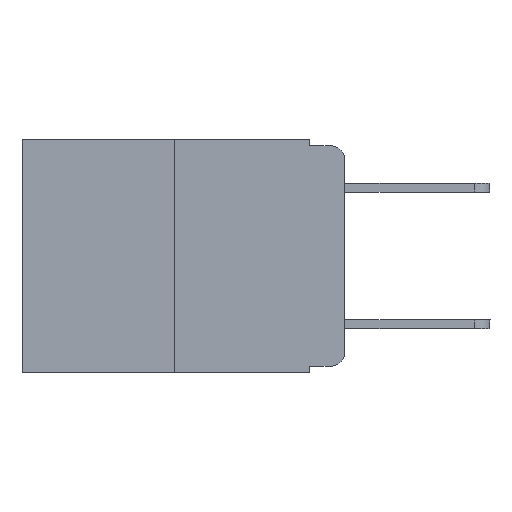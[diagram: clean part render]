
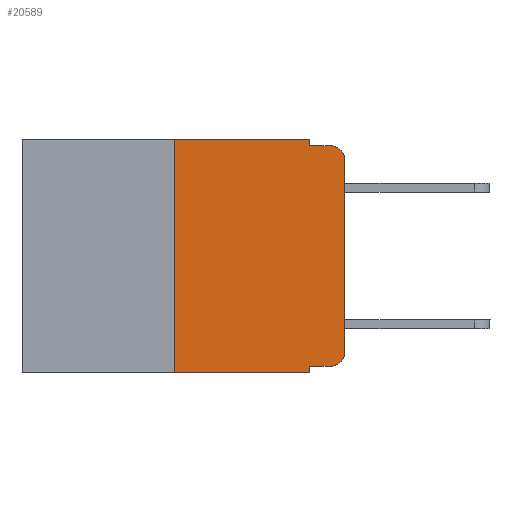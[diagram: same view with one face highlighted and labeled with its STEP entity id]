
A CAD part, left-side view. The second image highlights one B-rep face of the part: STEP entity #20589.
In plain terms, the highlighted planar face has unit normal (-1, 0, 0).
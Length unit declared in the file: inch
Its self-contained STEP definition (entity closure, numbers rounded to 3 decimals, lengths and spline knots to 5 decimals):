
#69 = DIRECTION ( 'NONE',  ( 0., 0., -1. ) ) ;
#441 = DIRECTION ( 'NONE',  ( 0., -1., 0. ) ) ;
#652 = EDGE_LOOP ( 'NONE', ( #15446, #8806, #4839, #7220, #18919, #14201, #16379, #14491, #13478, #13454 ) ) ;
#856 = CARTESIAN_POINT ( 'NONE',  ( 0., 0.473, 0. ) ) ;
#1182 = VERTEX_POINT ( 'NONE', #15359 ) ;
#1519 = VECTOR ( 'NONE', #8959, 39.37008 ) ;
#1958 = CARTESIAN_POINT ( 'NONE',  ( 0., 0.051, 0. ) ) ;
#2366 = VECTOR ( 'NONE', #7526, 39.37008 ) ;
#3283 = EDGE_CURVE ( 'NONE', #16413, #15530, #4092, .T. ) ;
#3313 = DIRECTION ( 'NONE',  ( 0., -1., 0. ) ) ;
#3747 = DIRECTION ( 'NONE',  ( 0., 0., 1. ) ) ;
#3876 = EDGE_CURVE ( 'NONE', #3995, #9396, #10970, .T. ) ;
#3995 = VERTEX_POINT ( 'NONE', #16240 ) ;
#4092 = CIRCLE ( 'NONE', #11874, 0.02 ) ;
#4710 = CARTESIAN_POINT ( 'NONE',  ( 0., 0.02, -0.333 ) ) ;
#4839 = ORIENTED_EDGE ( 'NONE', *, *, #11052, .F. ) ;
#5155 = CARTESIAN_POINT ( 'NONE',  ( 0., 0., -0.313 ) ) ;
#5842 = DIRECTION ( 'NONE',  ( -1., 0., 0. ) ) ;
#6156 = VECTOR ( 'NONE', #3747, 39.37008 ) ;
#6879 = EDGE_CURVE ( 'NONE', #3995, #14128, #8484, .T. ) ;
#6946 = DIRECTION ( 'NONE',  ( 0., 0., 1. ) ) ;
#7149 = VECTOR ( 'NONE', #3313, 39.37008 ) ;
#7220 = ORIENTED_EDGE ( 'NONE', *, *, #13055, .F. ) ;
#7289 = VECTOR ( 'NONE', #6946, 39.37008 ) ;
#7526 = DIRECTION ( 'NONE',  ( 0., -1., 0. ) ) ;
#7574 = AXIS2_PLACEMENT_3D ( 'NONE', #856, #13953, #9022 ) ;
#7585 = CARTESIAN_POINT ( 'NONE',  ( 0., 0.051, -0.343 ) ) ;
#7657 = EDGE_CURVE ( 'NONE', #13780, #16413, #10781, .T. ) ;
#7658 = CARTESIAN_POINT ( 'NONE',  ( 0., 0.051, 0. ) ) ;
#8283 = CARTESIAN_POINT ( 'NONE',  ( 0., 0.051, -0.01 ) ) ;
#8305 = CARTESIAN_POINT ( 'NONE',  ( 0., 0.473, -0.343 ) ) ;
#8444 = DIRECTION ( 'NONE',  ( 0., 0., -1. ) ) ;
#8484 = LINE ( 'NONE', #12313, #2366 ) ;
#8601 = CARTESIAN_POINT ( 'NONE',  ( 0., 0.473, 0. ) ) ;
#8806 = ORIENTED_EDGE ( 'NONE', *, *, #3283, .T. ) ;
#8959 = DIRECTION ( 'NONE',  ( 0., 0., -1. ) ) ;
#9022 = DIRECTION ( 'NONE',  ( 0., 0., -1. ) ) ;
#9098 = CARTESIAN_POINT ( 'NONE',  ( 0., 0.051, 0. ) ) ;
#9131 = CARTESIAN_POINT ( 'NONE',  ( 0., 0.25, 0. ) ) ;
#9346 = DIRECTION ( 'NONE',  ( 0., 0., -1. ) ) ;
#9396 = VERTEX_POINT ( 'NONE', #7585 ) ;
#9436 = VERTEX_POINT ( 'NONE', #7658 ) ;
#9834 = VECTOR ( 'NONE', #441, 39.37008 ) ;
#10781 = LINE ( 'NONE', #11898, #6156 ) ;
#10970 = LINE ( 'NONE', #9098, #1519 ) ;
#11025 = VERTEX_POINT ( 'NONE', #9131 ) ;
#11052 = EDGE_CURVE ( 'NONE', #15637, #15530, #18633, .T. ) ;
#11369 = EDGE_CURVE ( 'NONE', #1182, #11025, #18310, .T. ) ;
#11557 = CARTESIAN_POINT ( 'NONE',  ( 0., 0., -0.03 ) ) ;
#11560 = VECTOR ( 'NONE', #8444, 39.37008 ) ;
#11874 = AXIS2_PLACEMENT_3D ( 'NONE', #20680, #5842, #9346 ) ;
#11898 = CARTESIAN_POINT ( 'NONE',  ( 0., 0., 0. ) ) ;
#12313 = CARTESIAN_POINT ( 'NONE',  ( 0., 0.051, -0.333 ) ) ;
#12386 = PLANE ( 'NONE',  #7574 ) ;
#12904 = CARTESIAN_POINT ( 'NONE',  ( 0., 0.02, -0.313 ) ) ;
#13055 = EDGE_CURVE ( 'NONE', #9436, #15637, #18232, .T. ) ;
#13454 = ORIENTED_EDGE ( 'NONE', *, *, #16793, .T. ) ;
#13478 = ORIENTED_EDGE ( 'NONE', *, *, #6879, .T. ) ;
#13780 = VERTEX_POINT ( 'NONE', #5155 ) ;
#13922 = CARTESIAN_POINT ( 'NONE',  ( 0., 0.051, -0.01 ) ) ;
#13953 = DIRECTION ( 'NONE',  ( 1., 0., 0. ) ) ;
#13965 = AXIS2_PLACEMENT_3D ( 'NONE', #12904, #19734, #69 ) ;
#14128 = VERTEX_POINT ( 'NONE', #4710 ) ;
#14175 = LINE ( 'NONE', #8601, #9834 ) ;
#14201 = ORIENTED_EDGE ( 'NONE', *, *, #11369, .F. ) ;
#14491 = ORIENTED_EDGE ( 'NONE', *, *, #3876, .F. ) ;
#15027 = EDGE_CURVE ( 'NONE', #1182, #9396, #17666, .T. ) ;
#15249 = CARTESIAN_POINT ( 'NONE',  ( 0., 0.25, 0. ) ) ;
#15359 = CARTESIAN_POINT ( 'NONE',  ( 0., 0.25, -0.343 ) ) ;
#15446 = ORIENTED_EDGE ( 'NONE', *, *, #7657, .T. ) ;
#15530 = VERTEX_POINT ( 'NONE', #17851 ) ;
#15637 = VERTEX_POINT ( 'NONE', #8283 ) ;
#15855 = FACE_OUTER_BOUND ( 'NONE', #652, .T. ) ;
#16240 = CARTESIAN_POINT ( 'NONE',  ( 0., 0.051, -0.333 ) ) ;
#16379 = ORIENTED_EDGE ( 'NONE', *, *, #15027, .T. ) ;
#16413 = VERTEX_POINT ( 'NONE', #11557 ) ;
#16793 = EDGE_CURVE ( 'NONE', #14128, #13780, #20668, .T. ) ;
#17666 = LINE ( 'NONE', #8305, #7149 ) ;
#17851 = CARTESIAN_POINT ( 'NONE',  ( 0., 0.02, -0.01 ) ) ;
#18113 = VECTOR ( 'NONE', #18693, 39.37008 ) ;
#18232 = LINE ( 'NONE', #1958, #11560 ) ;
#18310 = LINE ( 'NONE', #15249, #7289 ) ;
#18503 = EDGE_CURVE ( 'NONE', #11025, #9436, #14175, .T. ) ;
#18633 = LINE ( 'NONE', #13922, #18113 ) ;
#18693 = DIRECTION ( 'NONE',  ( 0., -1., 0. ) ) ;
#18919 = ORIENTED_EDGE ( 'NONE', *, *, #18503, .F. ) ;
#19734 = DIRECTION ( 'NONE',  ( -1., 0., 0. ) ) ;
#20589 = ADVANCED_FACE ( 'NONE', ( #15855 ), #12386, .F. ) ;
#20668 = CIRCLE ( 'NONE', #13965, 0.02 ) ;
#20680 = CARTESIAN_POINT ( 'NONE',  ( 0., 0.02, -0.03 ) ) ;
